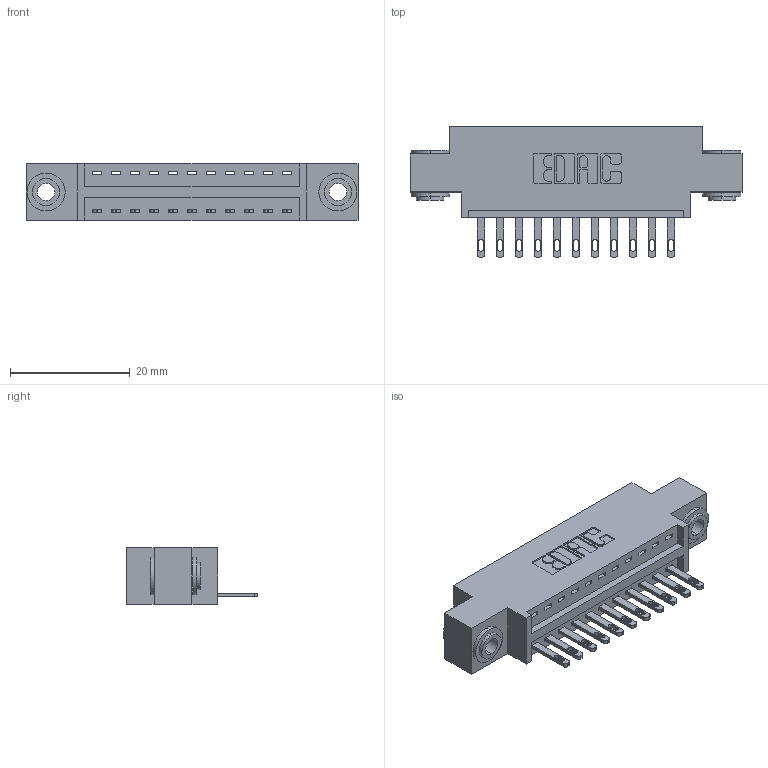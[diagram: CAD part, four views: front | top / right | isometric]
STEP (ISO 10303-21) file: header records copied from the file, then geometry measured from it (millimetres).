
FILE_DESCRIPTION (( 'STEP AP203' ), '1' );
FILE_NAME ('346-011-500-603.STEP', '2022-05-05T00:38:43', ( '' ), ( '' ), 'SwSTEP 2.0', 'SolidWorks 2020', '' );
FILE_SCHEMA (( 'CONFIG_CONTROL_DESIGN' ));
Length unit declared in the file: inch
Products named in the file (4): 345-250-002_345-250-002-102; 346-011-500-603; 346 Part_0.170 Offset - 0.156 Dia-TH; 345-292-001_345-293-100
Assembly tree (14 placements, depth 2):
  346-011-500-603
    346 Part_0.170 Offset - 0.156 Dia-TH
    345-292-001_345-293-100  x11
    345-250-002_345-250-002-102  x2
Bounding box: 55.5 x 21.84 x 9.4 mm (x, y, z)
Volume: 4952.4 mm3; surface area: 6292.8 mm2
Topology: 14 solids, 14 shells, 772 faces, 2301 edges, 1530 vertices
Faces by surface type: plane 478, cylinder 286, cone 8
Entity records: 12128 total; most frequent: CARTESIAN_POINT 2070, ORIENTED_EDGE 2006, DIRECTION 1895, EDGE_CURVE 1003, VECTOR 799, LINE 799, VERTEX_POINT 666, AXIS2_PLACEMENT_3D 548
